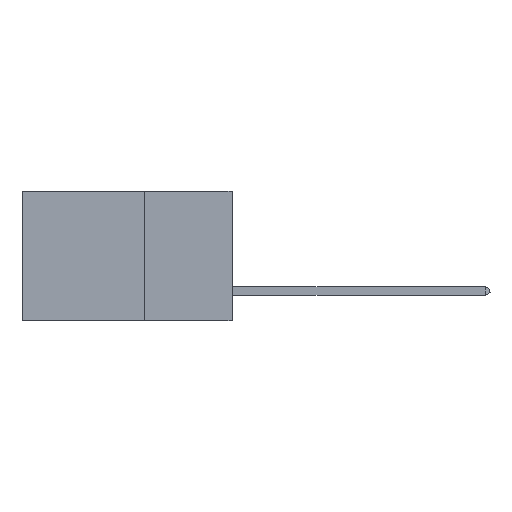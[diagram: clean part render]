
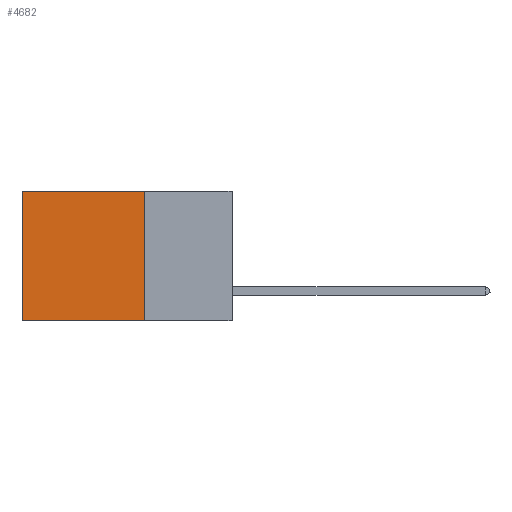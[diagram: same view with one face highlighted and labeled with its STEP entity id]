
A CAD part, left-side view. The second image highlights one B-rep face of the part: STEP entity #4682.
In plain terms, the highlighted planar face has unit normal (-1, 0, 0).
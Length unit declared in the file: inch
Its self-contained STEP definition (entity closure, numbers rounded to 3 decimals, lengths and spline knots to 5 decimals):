
#224 = CARTESIAN_POINT ( 'NONE',  ( 0.2875, 0.25, -0.37 ) ) ;
#1389 = LINE ( 'NONE', #10569, #10103 ) ;
#1839 = EDGE_CURVE ( 'NONE', #45769, #15051, #13436, .T. ) ;
#3035 = AXIS2_PLACEMENT_3D ( 'NONE', #15070, #18842, #44909 ) ;
#3526 = VECTOR ( 'NONE', #15504, 39.37008 ) ;
#4682 = ADVANCED_FACE ( 'NONE', ( #38923 ), #19327, .F. ) ;
#6485 = ORIENTED_EDGE ( 'NONE', *, *, #40276, .T. ) ;
#7664 = CARTESIAN_POINT ( 'NONE',  ( 0.2875, 0.6, 0. ) ) ;
#8222 = DIRECTION ( 'NONE',  ( 0., 0., -1. ) ) ;
#10103 = VECTOR ( 'NONE', #25647, 39.37008 ) ;
#10569 = CARTESIAN_POINT ( 'NONE',  ( 0.2875, 0.25, -0.37 ) ) ;
#11664 = CARTESIAN_POINT ( 'NONE',  ( 0.2875, 0.6, 0. ) ) ;
#13436 = LINE ( 'NONE', #21514, #3526 ) ;
#14620 = CARTESIAN_POINT ( 'NONE',  ( 0.2875, 0.6, -0.37 ) ) ;
#15051 = VERTEX_POINT ( 'NONE', #224 ) ;
#15070 = CARTESIAN_POINT ( 'NONE',  ( 0.2875, 0.25, 0. ) ) ;
#15504 = DIRECTION ( 'NONE',  ( 0., 0., -1. ) ) ;
#15685 = DIRECTION ( 'NONE',  ( 0., 1., 0. ) ) ;
#16494 = CARTESIAN_POINT ( 'NONE',  ( 0.2875, 0.25, 0. ) ) ;
#17367 = EDGE_LOOP ( 'NONE', ( #19489, #26265, #20538, #6485 ) ) ;
#18842 = DIRECTION ( 'NONE',  ( 1., 0., 0. ) ) ;
#18907 = EDGE_CURVE ( 'NONE', #37493, #36099, #22488, .T. ) ;
#19327 = PLANE ( 'NONE',  #3035 ) ;
#19489 = ORIENTED_EDGE ( 'NONE', *, *, #18907, .T. ) ;
#20538 = ORIENTED_EDGE ( 'NONE', *, *, #1839, .F. ) ;
#21514 = CARTESIAN_POINT ( 'NONE',  ( 0.2875, 0.25, 0. ) ) ;
#22488 = LINE ( 'NONE', #11664, #43444 ) ;
#25647 = DIRECTION ( 'NONE',  ( 0., 1., 0. ) ) ;
#26265 = ORIENTED_EDGE ( 'NONE', *, *, #44443, .F. ) ;
#30574 = LINE ( 'NONE', #30590, #39808 ) ;
#30590 = CARTESIAN_POINT ( 'NONE',  ( 0.2875, 0.25, 0. ) ) ;
#36099 = VERTEX_POINT ( 'NONE', #14620 ) ;
#37493 = VERTEX_POINT ( 'NONE', #7664 ) ;
#38923 = FACE_OUTER_BOUND ( 'NONE', #17367, .T. ) ;
#39808 = VECTOR ( 'NONE', #15685, 39.37008 ) ;
#40276 = EDGE_CURVE ( 'NONE', #45769, #37493, #30574, .T. ) ;
#43444 = VECTOR ( 'NONE', #8222, 39.37008 ) ;
#44443 = EDGE_CURVE ( 'NONE', #15051, #36099, #1389, .T. ) ;
#44909 = DIRECTION ( 'NONE',  ( 0., 0., -1. ) ) ;
#45769 = VERTEX_POINT ( 'NONE', #16494 ) ;
